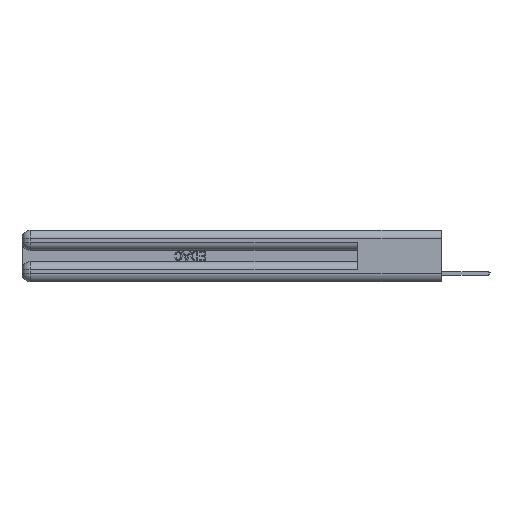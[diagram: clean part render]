
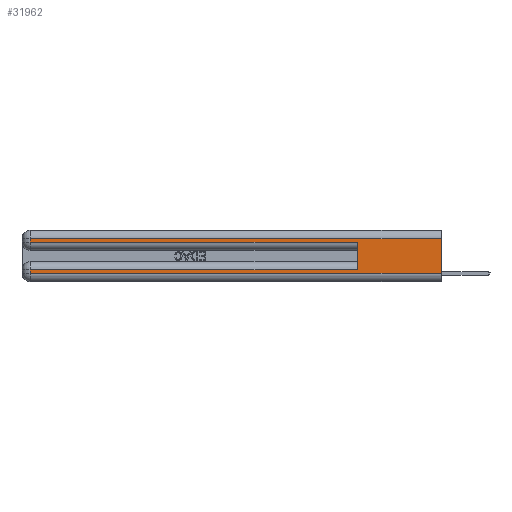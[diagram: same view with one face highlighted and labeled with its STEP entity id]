
A CAD part, left-side view. The second image highlights one B-rep face of the part: STEP entity #31962.
In plain terms, the highlighted planar face has unit normal (-1, 0, 0).
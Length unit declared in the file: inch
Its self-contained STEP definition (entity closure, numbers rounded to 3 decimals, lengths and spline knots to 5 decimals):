
#94 = VERTEX_POINT ( 'NONE', #7372 ) ;
#424 = ORIENTED_EDGE ( 'NONE', *, *, #27585, .F. ) ;
#743 = CARTESIAN_POINT ( 'NONE',  ( 0., 2.94, 0.06 ) ) ;
#773 = VERTEX_POINT ( 'NONE', #14741 ) ;
#1399 = EDGE_CURVE ( 'NONE', #1468, #23195, #10124, .T. ) ;
#1468 = VERTEX_POINT ( 'NONE', #31536 ) ;
#1561 = AXIS2_PLACEMENT_3D ( 'NONE', #21734, #6920, #14087 ) ;
#2577 = VECTOR ( 'NONE', #18487, 39.37008 ) ;
#2942 = EDGE_CURVE ( 'NONE', #9346, #6956, #17909, .T. ) ;
#3276 = EDGE_LOOP ( 'NONE', ( #424, #7768, #33481, #25950, #14697, #19452, #27049, #6582 ) ) ;
#4353 = DIRECTION ( 'NONE',  ( 0., 0., -1. ) ) ;
#6376 = VECTOR ( 'NONE', #4353, 39.37008 ) ;
#6582 = ORIENTED_EDGE ( 'NONE', *, *, #10159, .T. ) ;
#6920 = DIRECTION ( 'NONE',  ( 1., 0., 0. ) ) ;
#6956 = VERTEX_POINT ( 'NONE', #31799 ) ;
#7372 = CARTESIAN_POINT ( 'NONE',  ( 0., 2.94, 0.085 ) ) ;
#7740 = LINE ( 'NONE', #20980, #31121 ) ;
#7768 = ORIENTED_EDGE ( 'NONE', *, *, #1399, .T. ) ;
#8493 = VERTEX_POINT ( 'NONE', #15292 ) ;
#8592 = LINE ( 'NONE', #16584, #17196 ) ;
#8654 = LINE ( 'NONE', #33130, #9799 ) ;
#9146 = VECTOR ( 'NONE', #18716, 39.37008 ) ;
#9346 = VERTEX_POINT ( 'NONE', #33470 ) ;
#9715 = VECTOR ( 'NONE', #11997, 39.37008 ) ;
#9799 = VECTOR ( 'NONE', #21569, 39.37008 ) ;
#10124 = LINE ( 'NONE', #20485, #9715 ) ;
#10159 = EDGE_CURVE ( 'NONE', #13852, #773, #15763, .T. ) ;
#10384 = EDGE_CURVE ( 'NONE', #94, #13852, #17268, .T. ) ;
#10976 = DIRECTION ( 'NONE',  ( 0., 0., -1. ) ) ;
#11997 = DIRECTION ( 'NONE',  ( 0., 1., 0. ) ) ;
#13852 = VERTEX_POINT ( 'NONE', #743 ) ;
#14087 = DIRECTION ( 'NONE',  ( 0., 0., -1. ) ) ;
#14346 = DIRECTION ( 'NONE',  ( 0., -1., 0. ) ) ;
#14697 = ORIENTED_EDGE ( 'NONE', *, *, #2942, .F. ) ;
#14741 = CARTESIAN_POINT ( 'NONE',  ( 0., 0., 0.06 ) ) ;
#14767 = EDGE_CURVE ( 'NONE', #9346, #94, #8654, .T. ) ;
#15292 = CARTESIAN_POINT ( 'NONE',  ( 0., 2.94, 0.285 ) ) ;
#15763 = LINE ( 'NONE', #28869, #2577 ) ;
#16584 = CARTESIAN_POINT ( 'NONE',  ( 0., 0., 0.37 ) ) ;
#16600 = CARTESIAN_POINT ( 'NONE',  ( 0., 2.94, 0.37 ) ) ;
#17196 = VECTOR ( 'NONE', #10976, 39.37008 ) ;
#17268 = LINE ( 'NONE', #16600, #6376 ) ;
#17909 = LINE ( 'NONE', #31498, #9146 ) ;
#18236 = CARTESIAN_POINT ( 'NONE',  ( 0., 2.94, 0.31 ) ) ;
#18487 = DIRECTION ( 'NONE',  ( 0., -1., 0. ) ) ;
#18716 = DIRECTION ( 'NONE',  ( 0., 0., 1. ) ) ;
#19436 = CARTESIAN_POINT ( 'NONE',  ( 0., 0., 0.285 ) ) ;
#19452 = ORIENTED_EDGE ( 'NONE', *, *, #14767, .T. ) ;
#20485 = CARTESIAN_POINT ( 'NONE',  ( 0., 0., 0.31 ) ) ;
#20666 = DIRECTION ( 'NONE',  ( 0., 0., -1. ) ) ;
#20802 = EDGE_CURVE ( 'NONE', #8493, #6956, #32736, .T. ) ;
#20980 = CARTESIAN_POINT ( 'NONE',  ( 0., 2.94, 0.37 ) ) ;
#21433 = EDGE_CURVE ( 'NONE', #23195, #8493, #7740, .T. ) ;
#21569 = DIRECTION ( 'NONE',  ( 0., 1., 0. ) ) ;
#21734 = CARTESIAN_POINT ( 'NONE',  ( 0., 0., 0.37 ) ) ;
#22002 = VECTOR ( 'NONE', #14346, 39.37008 ) ;
#23195 = VERTEX_POINT ( 'NONE', #18236 ) ;
#25950 = ORIENTED_EDGE ( 'NONE', *, *, #20802, .T. ) ;
#27049 = ORIENTED_EDGE ( 'NONE', *, *, #10384, .T. ) ;
#27585 = EDGE_CURVE ( 'NONE', #1468, #773, #8592, .T. ) ;
#28869 = CARTESIAN_POINT ( 'NONE',  ( 0., 0., 0.06 ) ) ;
#29565 = FACE_OUTER_BOUND ( 'NONE', #3276, .T. ) ;
#31121 = VECTOR ( 'NONE', #20666, 39.37008 ) ;
#31498 = CARTESIAN_POINT ( 'NONE',  ( 0., 0.6, 0.145 ) ) ;
#31536 = CARTESIAN_POINT ( 'NONE',  ( 0., 0., 0.31 ) ) ;
#31799 = CARTESIAN_POINT ( 'NONE',  ( 0., 0.6, 0.285 ) ) ;
#31962 = ADVANCED_FACE ( 'NONE', ( #29565 ), #32298, .F. ) ;
#32298 = PLANE ( 'NONE',  #1561 ) ;
#32736 = LINE ( 'NONE', #19436, #22002 ) ;
#33130 = CARTESIAN_POINT ( 'NONE',  ( 0., 0., 0.085 ) ) ;
#33470 = CARTESIAN_POINT ( 'NONE',  ( 0., 0.6, 0.085 ) ) ;
#33481 = ORIENTED_EDGE ( 'NONE', *, *, #21433, .T. ) ;
